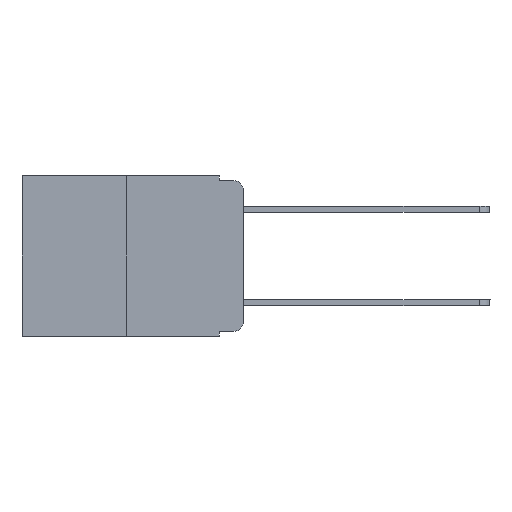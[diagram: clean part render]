
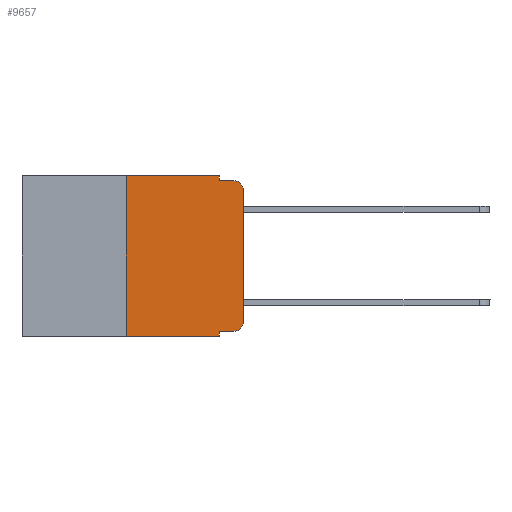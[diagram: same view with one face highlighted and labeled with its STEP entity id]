
A CAD part, left-side view. The second image highlights one B-rep face of the part: STEP entity #9657.
In plain terms, the highlighted planar face has unit normal (-1, 0, 0).
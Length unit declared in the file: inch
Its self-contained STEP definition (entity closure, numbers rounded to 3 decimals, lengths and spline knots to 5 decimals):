
#170 = CARTESIAN_POINT ( 'NONE',  ( 0., 0.051, -0.01 ) ) ;
#321 = DIRECTION ( 'NONE',  ( 0., 0., -1. ) ) ;
#356 = DIRECTION ( 'NONE',  ( 0., -1., 0. ) ) ;
#432 = CARTESIAN_POINT ( 'NONE',  ( 0., 0.051, -0.333 ) ) ;
#481 = CARTESIAN_POINT ( 'NONE',  ( 0., 0., 0. ) ) ;
#620 = VERTEX_POINT ( 'NONE', #4504 ) ;
#621 = VERTEX_POINT ( 'NONE', #432 ) ;
#650 = CARTESIAN_POINT ( 'NONE',  ( 0., 0.473, -0.343 ) ) ;
#912 = LINE ( 'NONE', #170, #2959 ) ;
#1039 = LINE ( 'NONE', #7185, #12798 ) ;
#1193 = VERTEX_POINT ( 'NONE', #5500 ) ;
#1214 = DIRECTION ( 'NONE',  ( 0., -1., 0. ) ) ;
#1456 = VERTEX_POINT ( 'NONE', #12137 ) ;
#1476 = EDGE_CURVE ( 'NONE', #621, #12095, #11298, .T. ) ;
#1788 = VERTEX_POINT ( 'NONE', #4644 ) ;
#2169 = CARTESIAN_POINT ( 'NONE',  ( 0., 0.02, -0.313 ) ) ;
#2377 = DIRECTION ( 'NONE',  ( -1., 0., 0. ) ) ;
#2635 = VECTOR ( 'NONE', #9770, 39.37008 ) ;
#2747 = AXIS2_PLACEMENT_3D ( 'NONE', #9122, #3928, #9958 ) ;
#2959 = VECTOR ( 'NONE', #1214, 39.37008 ) ;
#3091 = LINE ( 'NONE', #8788, #10910 ) ;
#3148 = EDGE_CURVE ( 'NONE', #1788, #10425, #5807, .T. ) ;
#3225 = EDGE_CURVE ( 'NONE', #620, #10018, #8372, .T. ) ;
#3734 = VERTEX_POINT ( 'NONE', #11155 ) ;
#3928 = DIRECTION ( 'NONE',  ( 1., 0., 0. ) ) ;
#4504 = CARTESIAN_POINT ( 'NONE',  ( 0., 0., -0.03 ) ) ;
#4549 = ORIENTED_EDGE ( 'NONE', *, *, #8951, .T. ) ;
#4644 = CARTESIAN_POINT ( 'NONE',  ( 0., 0.25, 0. ) ) ;
#4829 = VECTOR ( 'NONE', #11160, 39.37008 ) ;
#5385 = VECTOR ( 'NONE', #8655, 39.37008 ) ;
#5500 = CARTESIAN_POINT ( 'NONE',  ( 0., 0., -0.313 ) ) ;
#5661 = CARTESIAN_POINT ( 'NONE',  ( 0., 0.25, 0. ) ) ;
#5792 = DIRECTION ( 'NONE',  ( 0., -1., 0. ) ) ;
#5807 = LINE ( 'NONE', #11849, #4829 ) ;
#6002 = DIRECTION ( 'NONE',  ( -1., 0., 0. ) ) ;
#6109 = ORIENTED_EDGE ( 'NONE', *, *, #1476, .F. ) ;
#6406 = ORIENTED_EDGE ( 'NONE', *, *, #11929, .F. ) ;
#6564 = ORIENTED_EDGE ( 'NONE', *, *, #3225, .T. ) ;
#6839 = CARTESIAN_POINT ( 'NONE',  ( 0., 0.02, -0.01 ) ) ;
#6898 = ORIENTED_EDGE ( 'NONE', *, *, #12510, .T. ) ;
#7019 = CARTESIAN_POINT ( 'NONE',  ( 0., 0.02, -0.03 ) ) ;
#7138 = EDGE_LOOP ( 'NONE', ( #13177, #6564, #12864, #11292, #12499, #6406, #4549, #6109, #6898, #12138 ) ) ;
#7185 = CARTESIAN_POINT ( 'NONE',  ( 0., 0.051, 0. ) ) ;
#7693 = EDGE_CURVE ( 'NONE', #1456, #1193, #10267, .T. ) ;
#8179 = VECTOR ( 'NONE', #356, 39.37008 ) ;
#8372 = CIRCLE ( 'NONE', #10046, 0.02 ) ;
#8655 = DIRECTION ( 'NONE',  ( 0., 0., 1. ) ) ;
#8696 = VERTEX_POINT ( 'NONE', #12949 ) ;
#8788 = CARTESIAN_POINT ( 'NONE',  ( 0., 0.051, -0.333 ) ) ;
#8951 = EDGE_CURVE ( 'NONE', #3734, #12095, #10859, .T. ) ;
#9054 = LINE ( 'NONE', #5661, #2635 ) ;
#9122 = CARTESIAN_POINT ( 'NONE',  ( 0., 0.473, 0. ) ) ;
#9657 = ADVANCED_FACE ( 'NONE', ( #10830 ), #10927, .F. ) ;
#9770 = DIRECTION ( 'NONE',  ( 0., 0., 1. ) ) ;
#9958 = DIRECTION ( 'NONE',  ( 0., 0., -1. ) ) ;
#10018 = VERTEX_POINT ( 'NONE', #6839 ) ;
#10046 = AXIS2_PLACEMENT_3D ( 'NONE', #7019, #6002, #13245 ) ;
#10267 = CIRCLE ( 'NONE', #10672, 0.02 ) ;
#10425 = VERTEX_POINT ( 'NONE', #10532 ) ;
#10532 = CARTESIAN_POINT ( 'NONE',  ( 0., 0.051, 0. ) ) ;
#10545 = EDGE_CURVE ( 'NONE', #1193, #620, #12553, .T. ) ;
#10672 = AXIS2_PLACEMENT_3D ( 'NONE', #2169, #2377, #321 ) ;
#10830 = FACE_OUTER_BOUND ( 'NONE', #7138, .T. ) ;
#10859 = LINE ( 'NONE', #650, #8179 ) ;
#10910 = VECTOR ( 'NONE', #5792, 39.37008 ) ;
#10927 = PLANE ( 'NONE',  #2747 ) ;
#11114 = DIRECTION ( 'NONE',  ( 0., 0., -1. ) ) ;
#11155 = CARTESIAN_POINT ( 'NONE',  ( 0., 0.25, -0.343 ) ) ;
#11160 = DIRECTION ( 'NONE',  ( 0., -1., 0. ) ) ;
#11292 = ORIENTED_EDGE ( 'NONE', *, *, #11534, .F. ) ;
#11298 = LINE ( 'NONE', #12045, #13060 ) ;
#11534 = EDGE_CURVE ( 'NONE', #10425, #8696, #1039, .T. ) ;
#11710 = EDGE_CURVE ( 'NONE', #8696, #10018, #912, .T. ) ;
#11849 = CARTESIAN_POINT ( 'NONE',  ( 0., 0.473, 0. ) ) ;
#11929 = EDGE_CURVE ( 'NONE', #3734, #1788, #9054, .T. ) ;
#12045 = CARTESIAN_POINT ( 'NONE',  ( 0., 0.051, 0. ) ) ;
#12095 = VERTEX_POINT ( 'NONE', #12116 ) ;
#12116 = CARTESIAN_POINT ( 'NONE',  ( 0., 0.051, -0.343 ) ) ;
#12137 = CARTESIAN_POINT ( 'NONE',  ( 0., 0.02, -0.333 ) ) ;
#12138 = ORIENTED_EDGE ( 'NONE', *, *, #7693, .T. ) ;
#12499 = ORIENTED_EDGE ( 'NONE', *, *, #3148, .F. ) ;
#12510 = EDGE_CURVE ( 'NONE', #621, #1456, #3091, .T. ) ;
#12553 = LINE ( 'NONE', #481, #5385 ) ;
#12798 = VECTOR ( 'NONE', #11114, 39.37008 ) ;
#12864 = ORIENTED_EDGE ( 'NONE', *, *, #11710, .F. ) ;
#12949 = CARTESIAN_POINT ( 'NONE',  ( 0., 0.051, -0.01 ) ) ;
#13049 = DIRECTION ( 'NONE',  ( 0., 0., -1. ) ) ;
#13060 = VECTOR ( 'NONE', #13049, 39.37008 ) ;
#13177 = ORIENTED_EDGE ( 'NONE', *, *, #10545, .T. ) ;
#13245 = DIRECTION ( 'NONE',  ( 0., 0., -1. ) ) ;
